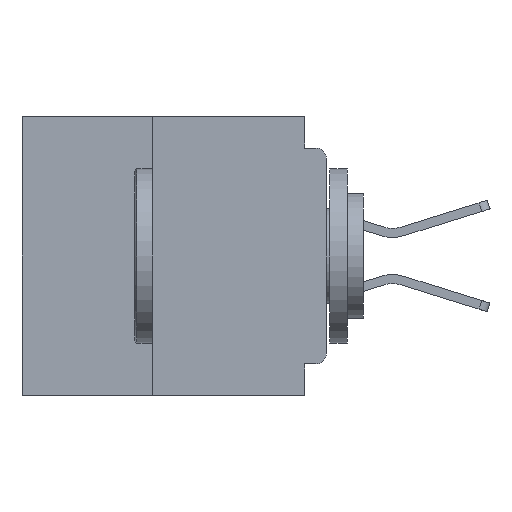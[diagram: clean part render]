
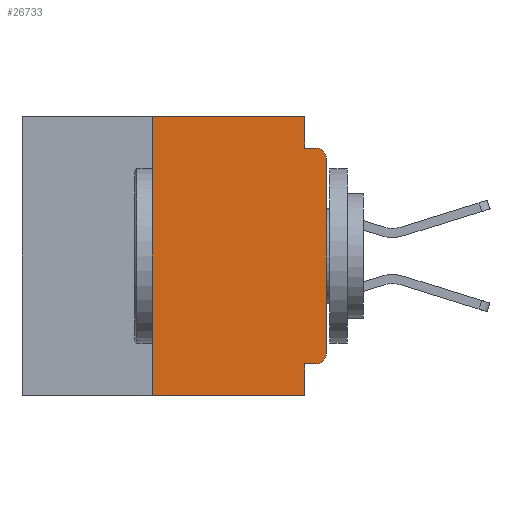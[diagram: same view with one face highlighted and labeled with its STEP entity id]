
A CAD part, left-side view. The second image highlights one B-rep face of the part: STEP entity #26733.
In plain terms, the highlighted planar face has unit normal (-1, 0, 0).
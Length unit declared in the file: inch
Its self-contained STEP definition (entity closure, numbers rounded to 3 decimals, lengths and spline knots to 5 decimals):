
#1010 = CARTESIAN_POINT ( 'NONE',  ( 0., 0.437, 0. ) ) ;
#1198 = DIRECTION ( 'NONE',  ( 0., 0., -1. ) ) ;
#1423 = EDGE_CURVE ( 'NONE', #46772, #51298, #13397, .T. ) ;
#1530 = EDGE_CURVE ( 'NONE', #45596, #44401, #16656, .T. ) ;
#2112 = CARTESIAN_POINT ( 'NONE',  ( 0., 0.031, -0.4 ) ) ;
#3062 = CIRCLE ( 'NONE', #18737, 0.015 ) ;
#3322 = EDGE_CURVE ( 'NONE', #14831, #43810, #7293, .T. ) ;
#3356 = ORIENTED_EDGE ( 'NONE', *, *, #28896, .F. ) ;
#5987 = VERTEX_POINT ( 'NONE', #48994 ) ;
#5994 = VECTOR ( 'NONE', #23843, 39.37008 ) ;
#6527 = CARTESIAN_POINT ( 'NONE',  ( 0., 0.015, -0.045 ) ) ;
#7110 = DIRECTION ( 'NONE',  ( 0., -1., 0. ) ) ;
#7139 = EDGE_CURVE ( 'NONE', #46772, #16412, #50505, .T. ) ;
#7171 = CARTESIAN_POINT ( 'NONE',  ( 0., 0., -0.045 ) ) ;
#7293 = LINE ( 'NONE', #7171, #51695 ) ;
#7374 = CARTESIAN_POINT ( 'NONE',  ( 0., 0.031, 0. ) ) ;
#7513 = CARTESIAN_POINT ( 'NONE',  ( 0., 0.015, -0.06 ) ) ;
#8841 = FACE_OUTER_BOUND ( 'NONE', #15515, .T. ) ;
#9253 = ORIENTED_EDGE ( 'NONE', *, *, #23114, .T. ) ;
#9999 = EDGE_CURVE ( 'NONE', #16269, #14831, #40314, .T. ) ;
#10550 = DIRECTION ( 'NONE',  ( 0., 0., 1. ) ) ;
#11794 = DIRECTION ( 'NONE',  ( 0., 0., -1. ) ) ;
#12823 = ORIENTED_EDGE ( 'NONE', *, *, #29696, .F. ) ;
#13397 = LINE ( 'NONE', #27990, #21930 ) ;
#14729 = DIRECTION ( 'NONE',  ( 0., 0., -1. ) ) ;
#14831 = VERTEX_POINT ( 'NONE', #41338 ) ;
#15429 = DIRECTION ( 'NONE',  ( 0., 0., -1. ) ) ;
#15515 = EDGE_LOOP ( 'NONE', ( #9253, #19042, #29450, #26027, #3356, #43674, #20405, #41838, #12823, #35231 ) ) ;
#15606 = DIRECTION ( 'NONE',  ( -1., 0., 0. ) ) ;
#15614 = CARTESIAN_POINT ( 'NONE',  ( 0., 0.015, -0.34 ) ) ;
#16269 = VERTEX_POINT ( 'NONE', #7374 ) ;
#16412 = VERTEX_POINT ( 'NONE', #16943 ) ;
#16656 = CIRCLE ( 'NONE', #35504, 0.015 ) ;
#16943 = CARTESIAN_POINT ( 'NONE',  ( 0., 0.25, 0. ) ) ;
#17120 = CARTESIAN_POINT ( 'NONE',  ( 0., 0.031, 0. ) ) ;
#17229 = LINE ( 'NONE', #48741, #5994 ) ;
#17514 = DIRECTION ( 'NONE',  ( 0., 0., 1. ) ) ;
#18323 = CARTESIAN_POINT ( 'NONE',  ( 0., 0.25, -0.4 ) ) ;
#18581 = EDGE_CURVE ( 'NONE', #5987, #43810, #3062, .T. ) ;
#18737 = AXIS2_PLACEMENT_3D ( 'NONE', #7513, #36737, #11794 ) ;
#19042 = ORIENTED_EDGE ( 'NONE', *, *, #18581, .T. ) ;
#19176 = LINE ( 'NONE', #42430, #31515 ) ;
#20405 = ORIENTED_EDGE ( 'NONE', *, *, #1423, .T. ) ;
#21930 = VECTOR ( 'NONE', #29056, 39.37008 ) ;
#23114 = EDGE_CURVE ( 'NONE', #44401, #5987, #19176, .T. ) ;
#23843 = DIRECTION ( 'NONE',  ( 0., -1., 0. ) ) ;
#26027 = ORIENTED_EDGE ( 'NONE', *, *, #9999, .F. ) ;
#26410 = DIRECTION ( 'NONE',  ( 1., 0., 0. ) ) ;
#26590 = CARTESIAN_POINT ( 'NONE',  ( 0., 0.015, -0.355 ) ) ;
#26733 = ADVANCED_FACE ( 'NONE', ( #8841 ), #51312, .F. ) ;
#26904 = LINE ( 'NONE', #31806, #37949 ) ;
#27076 = VECTOR ( 'NONE', #10550, 39.37008 ) ;
#27086 = CARTESIAN_POINT ( 'NONE',  ( 0., 0., -0.34 ) ) ;
#27990 = CARTESIAN_POINT ( 'NONE',  ( 0., 0.437, -0.4 ) ) ;
#28896 = EDGE_CURVE ( 'NONE', #16412, #16269, #17229, .T. ) ;
#29056 = DIRECTION ( 'NONE',  ( 0., -1., 0. ) ) ;
#29106 = LINE ( 'NONE', #2112, #38881 ) ;
#29243 = VECTOR ( 'NONE', #37853, 39.37008 ) ;
#29450 = ORIENTED_EDGE ( 'NONE', *, *, #3322, .F. ) ;
#29696 = EDGE_CURVE ( 'NONE', #45596, #34422, #26904, .T. ) ;
#31515 = VECTOR ( 'NONE', #17514, 39.37008 ) ;
#31806 = CARTESIAN_POINT ( 'NONE',  ( 0., 0., -0.355 ) ) ;
#34422 = VERTEX_POINT ( 'NONE', #46078 ) ;
#35231 = ORIENTED_EDGE ( 'NONE', *, *, #1530, .T. ) ;
#35504 = AXIS2_PLACEMENT_3D ( 'NONE', #15614, #15606, #15429 ) ;
#36737 = DIRECTION ( 'NONE',  ( -1., 0., 0. ) ) ;
#37853 = DIRECTION ( 'NONE',  ( 0., 0., -1. ) ) ;
#37949 = VECTOR ( 'NONE', #52531, 39.37008 ) ;
#38881 = VECTOR ( 'NONE', #14729, 39.37008 ) ;
#40314 = LINE ( 'NONE', #17120, #29243 ) ;
#41338 = CARTESIAN_POINT ( 'NONE',  ( 0., 0.031, -0.045 ) ) ;
#41838 = ORIENTED_EDGE ( 'NONE', *, *, #52921, .F. ) ;
#42430 = CARTESIAN_POINT ( 'NONE',  ( 0., 0., 0. ) ) ;
#43674 = ORIENTED_EDGE ( 'NONE', *, *, #7139, .F. ) ;
#43810 = VERTEX_POINT ( 'NONE', #6527 ) ;
#44401 = VERTEX_POINT ( 'NONE', #27086 ) ;
#45596 = VERTEX_POINT ( 'NONE', #26590 ) ;
#46078 = CARTESIAN_POINT ( 'NONE',  ( 0., 0.031, -0.355 ) ) ;
#46772 = VERTEX_POINT ( 'NONE', #18323 ) ;
#46847 = CARTESIAN_POINT ( 'NONE',  ( 0., 0.031, -0.4 ) ) ;
#47882 = CARTESIAN_POINT ( 'NONE',  ( 0., 0.25, -0.4 ) ) ;
#48741 = CARTESIAN_POINT ( 'NONE',  ( 0., 0.437, 0. ) ) ;
#48994 = CARTESIAN_POINT ( 'NONE',  ( 0., 0., -0.06 ) ) ;
#50505 = LINE ( 'NONE', #47882, #27076 ) ;
#51298 = VERTEX_POINT ( 'NONE', #46847 ) ;
#51312 = PLANE ( 'NONE',  #53790 ) ;
#51695 = VECTOR ( 'NONE', #7110, 39.37008 ) ;
#52531 = DIRECTION ( 'NONE',  ( 0., 1., 0. ) ) ;
#52921 = EDGE_CURVE ( 'NONE', #34422, #51298, #29106, .T. ) ;
#53790 = AXIS2_PLACEMENT_3D ( 'NONE', #1010, #26410, #1198 ) ;
